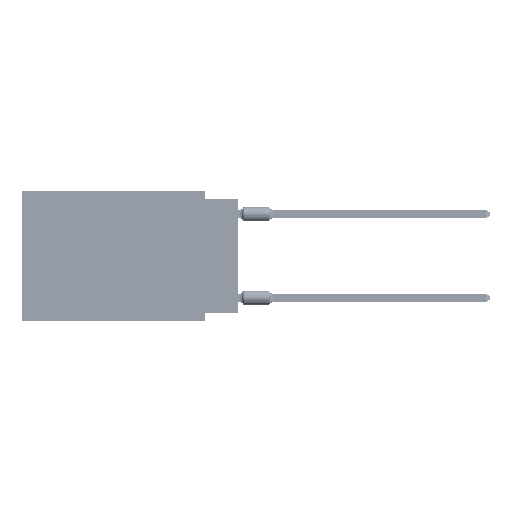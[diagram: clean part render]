
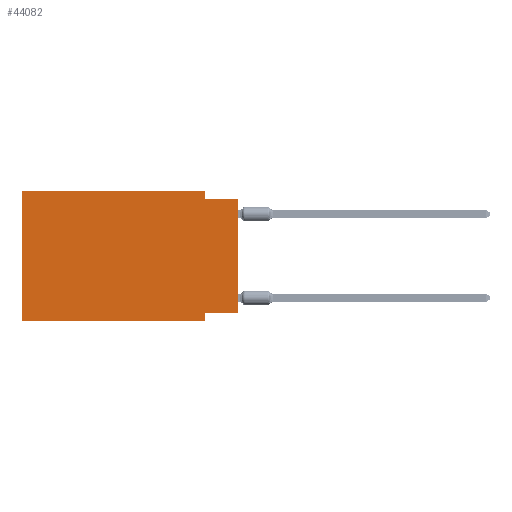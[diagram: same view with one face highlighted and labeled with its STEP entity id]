
A CAD part, left-side view. The second image highlights one B-rep face of the part: STEP entity #44082.
In plain terms, the highlighted planar face has unit normal (-1, 0, 0).
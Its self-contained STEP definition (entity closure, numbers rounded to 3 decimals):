
#823 = EDGE_CURVE ( 'NONE', #37878, #43195, #46482, .T. ) ;
#2498 = LINE ( 'NONE', #58430, #54045 ) ;
#4378 = EDGE_LOOP ( 'NONE', ( #67262, #38263, #41649, #36406, #62855, #51509, #12497, #12180 ) ) ;
#5626 = EDGE_CURVE ( 'NONE', #71097, #11179, #2498, .T. ) ;
#6623 = CARTESIAN_POINT ( 'NONE',  ( 0., 0., 0. ) ) ;
#7582 = DIRECTION ( 'NONE',  ( 0., 1., 0. ) ) ;
#11179 = VERTEX_POINT ( 'NONE', #25206 ) ;
#11370 = VECTOR ( 'NONE', #67122, 1000. ) ;
#12177 = VECTOR ( 'NONE', #30379, 1000. ) ;
#12180 = ORIENTED_EDGE ( 'NONE', *, *, #5626, .F. ) ;
#12497 = ORIENTED_EDGE ( 'NONE', *, *, #65707, .F. ) ;
#13305 = CARTESIAN_POINT ( 'NONE',  ( 0., 2.54, -9.906 ) ) ;
#13717 = DIRECTION ( 'NONE',  ( 0., 0., -1. ) ) ;
#15740 = LINE ( 'NONE', #32097, #20696 ) ;
#16675 = VERTEX_POINT ( 'NONE', #28975 ) ;
#20696 = VECTOR ( 'NONE', #13717, 1000. ) ;
#21658 = CARTESIAN_POINT ( 'NONE',  ( 0., 0., -9.271 ) ) ;
#22850 = EDGE_CURVE ( 'NONE', #16675, #41507, #33705, .T. ) ;
#23956 = CARTESIAN_POINT ( 'NONE',  ( 0., 0., -0.635 ) ) ;
#25206 = CARTESIAN_POINT ( 'NONE',  ( 0., 2.54, -9.271 ) ) ;
#26678 = CARTESIAN_POINT ( 'NONE',  ( 0., 16.383, 0. ) ) ;
#27495 = DIRECTION ( 'NONE',  ( 1., 0., 0. ) ) ;
#28429 = LINE ( 'NONE', #6623, #62912 ) ;
#28975 = CARTESIAN_POINT ( 'NONE',  ( 0., 16.383, -9.906 ) ) ;
#30379 = DIRECTION ( 'NONE',  ( 0., 0., -1. ) ) ;
#31600 = VECTOR ( 'NONE', #62827, 1000. ) ;
#31824 = CARTESIAN_POINT ( 'NONE',  ( 0., 16.383, 0. ) ) ;
#32097 = CARTESIAN_POINT ( 'NONE',  ( 0., 2.54, 0. ) ) ;
#33705 = LINE ( 'NONE', #51124, #11370 ) ;
#34831 = VECTOR ( 'NONE', #41190, 1000. ) ;
#35103 = VECTOR ( 'NONE', #65247, 1000. ) ;
#36406 = ORIENTED_EDGE ( 'NONE', *, *, #52584, .F. ) ;
#37284 = LINE ( 'NONE', #31824, #35103 ) ;
#37878 = VERTEX_POINT ( 'NONE', #48929 ) ;
#38263 = ORIENTED_EDGE ( 'NONE', *, *, #823, .F. ) ;
#39917 = EDGE_CURVE ( 'NONE', #16675, #48779, #51364, .T. ) ;
#41190 = DIRECTION ( 'NONE',  ( 0., -1., 0. ) ) ;
#41507 = VERTEX_POINT ( 'NONE', #26678 ) ;
#41649 = ORIENTED_EDGE ( 'NONE', *, *, #69675, .F. ) ;
#43195 = VERTEX_POINT ( 'NONE', #59312 ) ;
#44082 = ADVANCED_FACE ( 'NONE', ( #67451 ), #45289, .F. ) ;
#44774 = CARTESIAN_POINT ( 'NONE',  ( 0., 2.54, -9.906 ) ) ;
#45141 = DIRECTION ( 'NONE',  ( 0., 0., 1. ) ) ;
#45289 = PLANE ( 'NONE',  #53947 ) ;
#46279 = CARTESIAN_POINT ( 'NONE',  ( 0., 16.383, -9.906 ) ) ;
#46482 = LINE ( 'NONE', #23956, #31600 ) ;
#48779 = VERTEX_POINT ( 'NONE', #44774 ) ;
#48929 = CARTESIAN_POINT ( 'NONE',  ( 0., 2.54, -0.635 ) ) ;
#49655 = DIRECTION ( 'NONE',  ( 0., 0., -1. ) ) ;
#50133 = VERTEX_POINT ( 'NONE', #53817 ) ;
#51124 = CARTESIAN_POINT ( 'NONE',  ( 0., 16.383, 0. ) ) ;
#51364 = LINE ( 'NONE', #46279, #34831 ) ;
#51509 = ORIENTED_EDGE ( 'NONE', *, *, #39917, .T. ) ;
#52173 = LINE ( 'NONE', #13305, #12177 ) ;
#52584 = EDGE_CURVE ( 'NONE', #41507, #50133, #37284, .T. ) ;
#53817 = CARTESIAN_POINT ( 'NONE',  ( 0., 2.54, 0. ) ) ;
#53947 = AXIS2_PLACEMENT_3D ( 'NONE', #61986, #27495, #49655 ) ;
#54045 = VECTOR ( 'NONE', #7582, 1000. ) ;
#58430 = CARTESIAN_POINT ( 'NONE',  ( 0., 0., -9.271 ) ) ;
#59312 = CARTESIAN_POINT ( 'NONE',  ( 0., 0., -0.635 ) ) ;
#60651 = EDGE_CURVE ( 'NONE', #71097, #43195, #28429, .T. ) ;
#61986 = CARTESIAN_POINT ( 'NONE',  ( 0., 16.383, 0. ) ) ;
#62827 = DIRECTION ( 'NONE',  ( 0., -1., 0. ) ) ;
#62855 = ORIENTED_EDGE ( 'NONE', *, *, #22850, .F. ) ;
#62912 = VECTOR ( 'NONE', #45141, 1000. ) ;
#65247 = DIRECTION ( 'NONE',  ( 0., -1., 0. ) ) ;
#65707 = EDGE_CURVE ( 'NONE', #11179, #48779, #52173, .T. ) ;
#67122 = DIRECTION ( 'NONE',  ( 0., 0., 1. ) ) ;
#67262 = ORIENTED_EDGE ( 'NONE', *, *, #60651, .T. ) ;
#67451 = FACE_OUTER_BOUND ( 'NONE', #4378, .T. ) ;
#69675 = EDGE_CURVE ( 'NONE', #50133, #37878, #15740, .T. ) ;
#71097 = VERTEX_POINT ( 'NONE', #21658 ) ;
